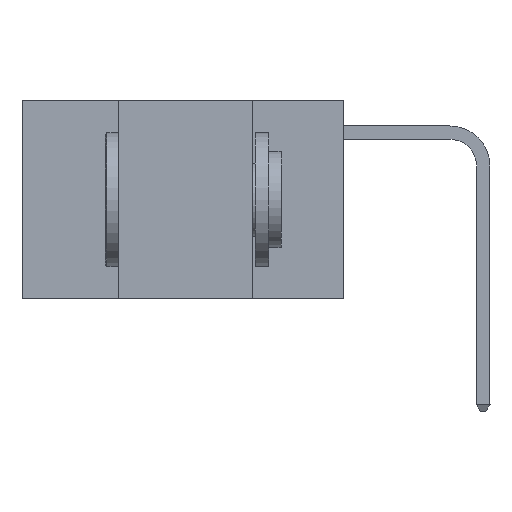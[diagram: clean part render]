
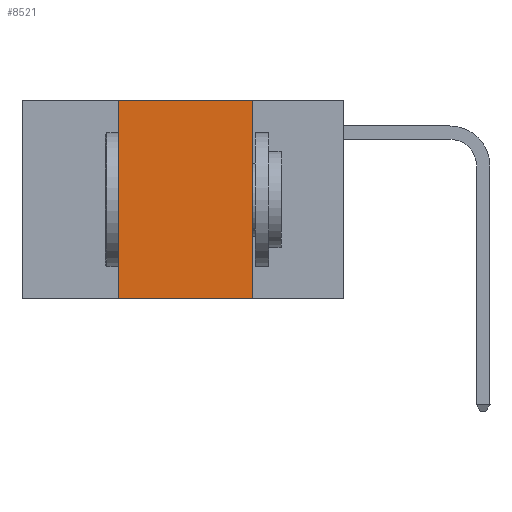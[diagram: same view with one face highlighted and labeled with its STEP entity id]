
A CAD part, left-side view. The second image highlights one B-rep face of the part: STEP entity #8521.
In plain terms, the highlighted planar face has unit normal (-1, 0, 0).
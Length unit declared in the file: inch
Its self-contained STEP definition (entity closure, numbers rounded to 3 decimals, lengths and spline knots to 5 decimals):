
#1988 = DIRECTION ( 'NONE',  ( 0., 0., 1. ) ) ;
#3019 = DIRECTION ( 'NONE',  ( 0., 0., -1. ) ) ;
#3571 = LINE ( 'NONE', #13194, #22058 ) ;
#3624 = VERTEX_POINT ( 'NONE', #19441 ) ;
#3735 = LINE ( 'NONE', #21153, #21708 ) ;
#4444 = LINE ( 'NONE', #14094, #17828 ) ;
#5512 = FACE_OUTER_BOUND ( 'NONE', #6723, .T. ) ;
#5670 = CARTESIAN_POINT ( 'NONE',  ( 0., 0.42, -0.37 ) ) ;
#6723 = EDGE_LOOP ( 'NONE', ( #9205, #18902, #15868, #9991 ) ) ;
#8158 = CARTESIAN_POINT ( 'NONE',  ( 0., 0.17, 0. ) ) ;
#8402 = EDGE_CURVE ( 'NONE', #19667, #3624, #3571, .T. ) ;
#8521 = ADVANCED_FACE ( 'NONE', ( #5512 ), #22110, .F. ) ;
#8798 = DIRECTION ( 'NONE',  ( 0., 0., -1. ) ) ;
#9205 = ORIENTED_EDGE ( 'NONE', *, *, #20081, .F. ) ;
#9760 = DIRECTION ( 'NONE',  ( 0., -1., 0. ) ) ;
#9991 = ORIENTED_EDGE ( 'NONE', *, *, #8402, .T. ) ;
#10770 = EDGE_CURVE ( 'NONE', #19667, #14161, #3735, .T. ) ;
#10886 = AXIS2_PLACEMENT_3D ( 'NONE', #11826, #13572, #3019 ) ;
#11095 = VERTEX_POINT ( 'NONE', #8158 ) ;
#11505 = CARTESIAN_POINT ( 'NONE',  ( 0., 0.6, 0. ) ) ;
#11826 = CARTESIAN_POINT ( 'NONE',  ( 0., 0.6, 0. ) ) ;
#12941 = EDGE_CURVE ( 'NONE', #14161, #11095, #17876, .T. ) ;
#13194 = CARTESIAN_POINT ( 'NONE',  ( 0., 0.6, -0.37 ) ) ;
#13288 = VECTOR ( 'NONE', #9760, 39.37008 ) ;
#13572 = DIRECTION ( 'NONE',  ( 1., 0., 0. ) ) ;
#14094 = CARTESIAN_POINT ( 'NONE',  ( 0., 0.17, 0. ) ) ;
#14161 = VERTEX_POINT ( 'NONE', #14764 ) ;
#14764 = CARTESIAN_POINT ( 'NONE',  ( 0., 0.42, 0. ) ) ;
#15868 = ORIENTED_EDGE ( 'NONE', *, *, #10770, .F. ) ;
#17828 = VECTOR ( 'NONE', #8798, 39.37008 ) ;
#17876 = LINE ( 'NONE', #11505, #13288 ) ;
#18423 = DIRECTION ( 'NONE',  ( 0., -1., 0. ) ) ;
#18902 = ORIENTED_EDGE ( 'NONE', *, *, #12941, .F. ) ;
#19441 = CARTESIAN_POINT ( 'NONE',  ( 0., 0.17, -0.37 ) ) ;
#19667 = VERTEX_POINT ( 'NONE', #5670 ) ;
#20081 = EDGE_CURVE ( 'NONE', #11095, #3624, #4444, .T. ) ;
#21153 = CARTESIAN_POINT ( 'NONE',  ( 0., 0.42, 0. ) ) ;
#21708 = VECTOR ( 'NONE', #1988, 39.37008 ) ;
#22058 = VECTOR ( 'NONE', #18423, 39.37008 ) ;
#22110 = PLANE ( 'NONE',  #10886 ) ;
